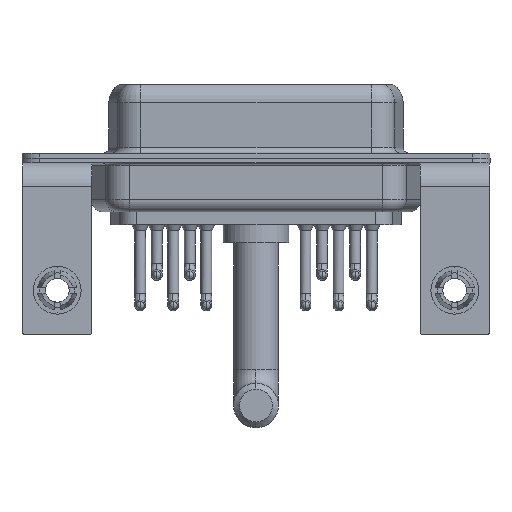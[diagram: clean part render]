
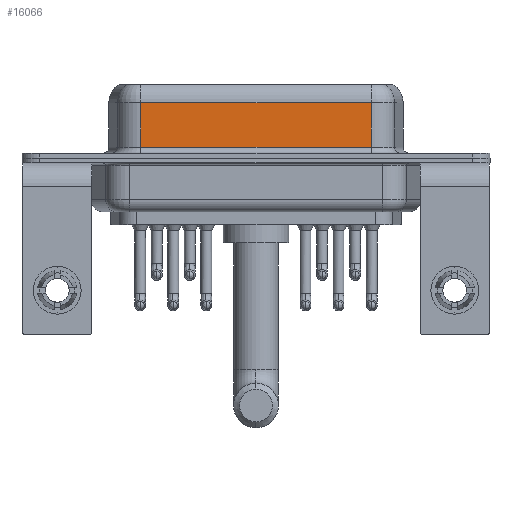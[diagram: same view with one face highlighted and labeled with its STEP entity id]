
A CAD part, front view. The second image highlights one B-rep face of the part: STEP entity #16066.
In plain terms, the highlighted planar face has unit normal (0, -1, 0).
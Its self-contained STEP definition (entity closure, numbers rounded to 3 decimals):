
#1329 = VECTOR ( 'NONE', #19468, 1000. ) ;
#1756 = DIRECTION ( 'NONE',  ( 0., 1., 0. ) ) ;
#2747 = ORIENTED_EDGE ( 'NONE', *, *, #14053, .T. ) ;
#3825 = LINE ( 'NONE', #10306, #5409 ) ;
#4491 = LINE ( 'NONE', #6503, #6394 ) ;
#4757 = LINE ( 'NONE', #14144, #18409 ) ;
#4959 = CARTESIAN_POINT ( 'NONE',  ( 7.013, -3.95, 6.4 ) ) ;
#5409 = VECTOR ( 'NONE', #8827, 1000. ) ;
#6054 = DIRECTION ( 'NONE',  ( -1., 0., 0. ) ) ;
#6394 = VECTOR ( 'NONE', #16199, 1000. ) ;
#6503 = CARTESIAN_POINT ( 'NONE',  ( 26.287, -3.95, 6.4 ) ) ;
#6642 = CARTESIAN_POINT ( 'NONE',  ( 26.287, -3.95, 6.4 ) ) ;
#6813 = CARTESIAN_POINT ( 'NONE',  ( 7.013, -3.95, 0.9 ) ) ;
#7183 = AXIS2_PLACEMENT_3D ( 'NONE', #6642, #1756, #18280 ) ;
#7822 = VERTEX_POINT ( 'NONE', #6813 ) ;
#8168 = ORIENTED_EDGE ( 'NONE', *, *, #13265, .F. ) ;
#8827 = DIRECTION ( 'NONE',  ( 1., 0., 0. ) ) ;
#9318 = EDGE_LOOP ( 'NONE', ( #8168, #9524, #20429, #2747 ) ) ;
#9524 = ORIENTED_EDGE ( 'NONE', *, *, #15405, .T. ) ;
#9619 = CARTESIAN_POINT ( 'NONE',  ( 7.013, -3.95, 4.65 ) ) ;
#9836 = FACE_OUTER_BOUND ( 'NONE', #9318, .T. ) ;
#9887 = CARTESIAN_POINT ( 'NONE',  ( 26.287, -3.95, 0.9 ) ) ;
#10306 = CARTESIAN_POINT ( 'NONE',  ( 26.287, -3.95, 0.9 ) ) ;
#11766 = VERTEX_POINT ( 'NONE', #9619 ) ;
#13265 = EDGE_CURVE ( 'NONE', #19919, #13917, #4491, .T. ) ;
#13917 = VERTEX_POINT ( 'NONE', #9887 ) ;
#14053 = EDGE_CURVE ( 'NONE', #7822, #13917, #3825, .T. ) ;
#14144 = CARTESIAN_POINT ( 'NONE',  ( 26.287, -3.95, 4.65 ) ) ;
#14284 = EDGE_CURVE ( 'NONE', #11766, #7822, #18196, .T. ) ;
#15405 = EDGE_CURVE ( 'NONE', #19919, #11766, #4757, .T. ) ;
#15696 = CARTESIAN_POINT ( 'NONE',  ( 26.287, -3.95, 4.65 ) ) ;
#16066 = ADVANCED_FACE ( 'NONE', ( #9836 ), #16337, .F. ) ;
#16199 = DIRECTION ( 'NONE',  ( 0., 0., -1. ) ) ;
#16337 = PLANE ( 'NONE',  #7183 ) ;
#18196 = LINE ( 'NONE', #4959, #1329 ) ;
#18280 = DIRECTION ( 'NONE',  ( 0., 0., 1. ) ) ;
#18409 = VECTOR ( 'NONE', #6054, 1000. ) ;
#19468 = DIRECTION ( 'NONE',  ( 0., 0., -1. ) ) ;
#19919 = VERTEX_POINT ( 'NONE', #15696 ) ;
#20429 = ORIENTED_EDGE ( 'NONE', *, *, #14284, .T. ) ;
